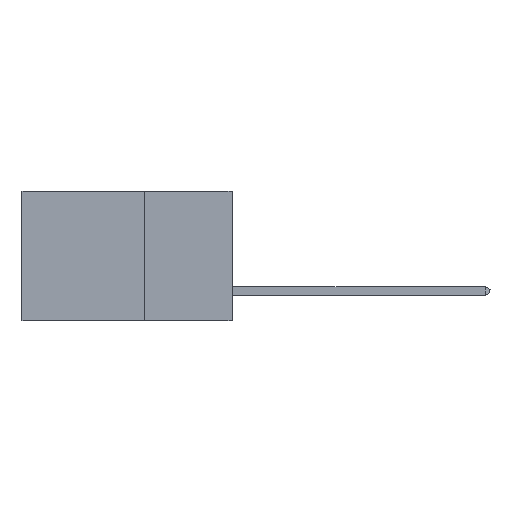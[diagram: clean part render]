
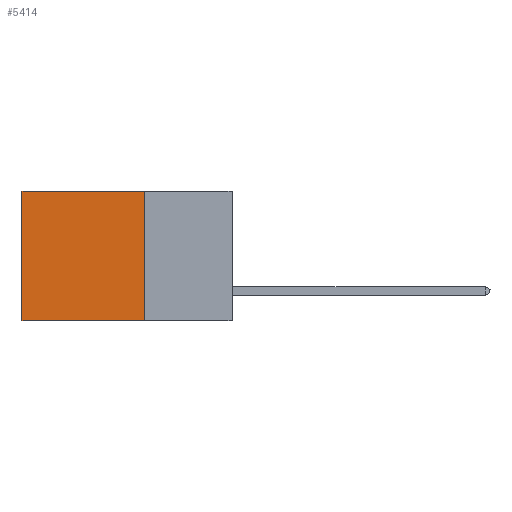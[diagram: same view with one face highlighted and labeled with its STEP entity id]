
A CAD part, left-side view. The second image highlights one B-rep face of the part: STEP entity #5414.
In plain terms, the highlighted planar face has unit normal (-1, 0, 0).
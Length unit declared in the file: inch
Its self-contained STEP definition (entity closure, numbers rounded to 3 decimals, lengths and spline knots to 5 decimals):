
#1076 = ORIENTED_EDGE ( 'NONE', *, *, #39772, .F. ) ;
#5080 = LINE ( 'NONE', #14744, #21739 ) ;
#5207 = EDGE_CURVE ( 'NONE', #11077, #37308, #41969, .T. ) ;
#5414 = ADVANCED_FACE ( 'NONE', ( #11083 ), #26057, .F. ) ;
#7234 = CARTESIAN_POINT ( 'NONE',  ( 0.2875, 0.25, 0. ) ) ;
#8467 = EDGE_LOOP ( 'NONE', ( #28226, #1076, #8753, #16707 ) ) ;
#8753 = ORIENTED_EDGE ( 'NONE', *, *, #33774, .F. ) ;
#8853 = AXIS2_PLACEMENT_3D ( 'NONE', #26902, #30803, #30975 ) ;
#10700 = LINE ( 'NONE', #26963, #21269 ) ;
#11077 = VERTEX_POINT ( 'NONE', #11326 ) ;
#11083 = FACE_OUTER_BOUND ( 'NONE', #8467, .T. ) ;
#11326 = CARTESIAN_POINT ( 'NONE',  ( 0.2875, 0.25, 0. ) ) ;
#14625 = DIRECTION ( 'NONE',  ( 0., 1., 0. ) ) ;
#14744 = CARTESIAN_POINT ( 'NONE',  ( 0.2875, 0.25, 0. ) ) ;
#15070 = CARTESIAN_POINT ( 'NONE',  ( 0.2875, 0.6, -0.37 ) ) ;
#16173 = VECTOR ( 'NONE', #34071, 39.37008 ) ;
#16707 = ORIENTED_EDGE ( 'NONE', *, *, #5207, .T. ) ;
#18850 = VERTEX_POINT ( 'NONE', #15070 ) ;
#20113 = DIRECTION ( 'NONE',  ( 0., 0., -1. ) ) ;
#21269 = VECTOR ( 'NONE', #20113, 39.37008 ) ;
#21739 = VECTOR ( 'NONE', #39802, 39.37008 ) ;
#22185 = VECTOR ( 'NONE', #14625, 39.37008 ) ;
#26057 = PLANE ( 'NONE',  #8853 ) ;
#26902 = CARTESIAN_POINT ( 'NONE',  ( 0.2875, 0.25, 0. ) ) ;
#26963 = CARTESIAN_POINT ( 'NONE',  ( 0.2875, 0.6, 0. ) ) ;
#28226 = ORIENTED_EDGE ( 'NONE', *, *, #42348, .T. ) ;
#28722 = VERTEX_POINT ( 'NONE', #36824 ) ;
#30094 = CARTESIAN_POINT ( 'NONE',  ( 0.2875, 0.6, 0. ) ) ;
#30745 = CARTESIAN_POINT ( 'NONE',  ( 0.2875, 0.25, -0.37 ) ) ;
#30803 = DIRECTION ( 'NONE',  ( 1., 0., 0. ) ) ;
#30975 = DIRECTION ( 'NONE',  ( 0., 0., -1. ) ) ;
#33774 = EDGE_CURVE ( 'NONE', #11077, #28722, #5080, .T. ) ;
#34071 = DIRECTION ( 'NONE',  ( 0., 1., 0. ) ) ;
#36824 = CARTESIAN_POINT ( 'NONE',  ( 0.2875, 0.25, -0.37 ) ) ;
#37308 = VERTEX_POINT ( 'NONE', #30094 ) ;
#37485 = LINE ( 'NONE', #30745, #16173 ) ;
#39772 = EDGE_CURVE ( 'NONE', #28722, #18850, #37485, .T. ) ;
#39802 = DIRECTION ( 'NONE',  ( 0., 0., -1. ) ) ;
#41969 = LINE ( 'NONE', #7234, #22185 ) ;
#42348 = EDGE_CURVE ( 'NONE', #37308, #18850, #10700, .T. ) ;
